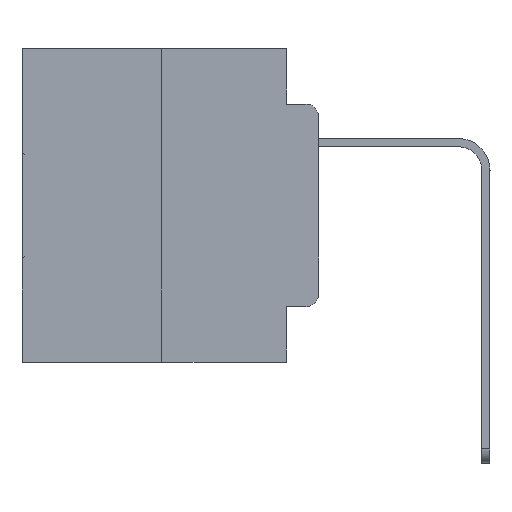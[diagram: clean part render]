
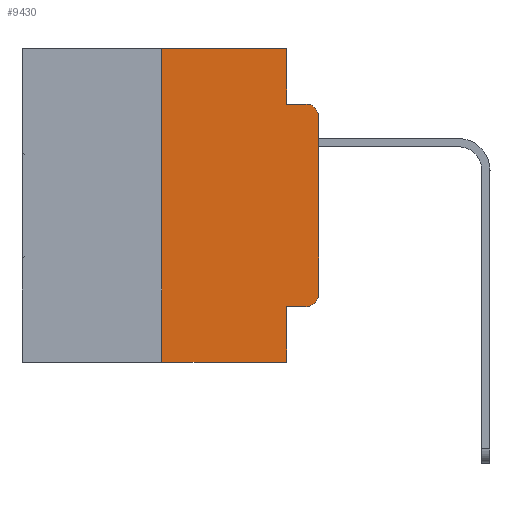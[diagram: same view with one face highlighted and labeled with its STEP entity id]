
A CAD part, left-side view. The second image highlights one B-rep face of the part: STEP entity #9430.
In plain terms, the highlighted planar face has unit normal (-1, 0, 0).
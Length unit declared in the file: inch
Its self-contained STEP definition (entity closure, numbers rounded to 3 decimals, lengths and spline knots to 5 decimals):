
#327 = ORIENTED_EDGE ( 'NONE', *, *, #11311, .F. ) ;
#585 = VECTOR ( 'NONE', #4701, 39.37008 ) ;
#1682 = CARTESIAN_POINT ( 'NONE',  ( 0., 0.473, -0.5 ) ) ;
#2079 = VERTEX_POINT ( 'NONE', #15576 ) ;
#2305 = VERTEX_POINT ( 'NONE', #29038 ) ;
#2365 = VERTEX_POINT ( 'NONE', #29349 ) ;
#2537 = AXIS2_PLACEMENT_3D ( 'NONE', #15377, #6257, #22660 ) ;
#2691 = CARTESIAN_POINT ( 'NONE',  ( 0., 0.473, 0. ) ) ;
#2839 = VERTEX_POINT ( 'NONE', #21788 ) ;
#3406 = CARTESIAN_POINT ( 'NONE',  ( 0., 0.02, -0.0885 ) ) ;
#3701 = DIRECTION ( 'NONE',  ( 0., 0., -1. ) ) ;
#3715 = CARTESIAN_POINT ( 'NONE',  ( 0., 0.25, 0. ) ) ;
#3877 = DIRECTION ( 'NONE',  ( 0., -1., 0. ) ) ;
#4158 = VERTEX_POINT ( 'NONE', #3406 ) ;
#4701 = DIRECTION ( 'NONE',  ( 0., -1., 0. ) ) ;
#4945 = ORIENTED_EDGE ( 'NONE', *, *, #18878, .F. ) ;
#5055 = CARTESIAN_POINT ( 'NONE',  ( 0., 0.25, 0. ) ) ;
#5182 = EDGE_CURVE ( 'NONE', #2079, #2305, #6317, .T. ) ;
#5239 = CARTESIAN_POINT ( 'NONE',  ( 0., 0.02, -0.4115 ) ) ;
#5759 = DIRECTION ( 'NONE',  ( 0., 0., 1. ) ) ;
#6077 = CARTESIAN_POINT ( 'NONE',  ( 0., 0., -0.3915 ) ) ;
#6252 = ORIENTED_EDGE ( 'NONE', *, *, #16830, .T. ) ;
#6257 = DIRECTION ( 'NONE',  ( -1., 0., 0. ) ) ;
#6317 = LINE ( 'NONE', #1682, #27460 ) ;
#6587 = CIRCLE ( 'NONE', #26185, 0.02 ) ;
#6698 = VECTOR ( 'NONE', #26611, 39.37008 ) ;
#6733 = CARTESIAN_POINT ( 'NONE',  ( 0., 0., -0.1085 ) ) ;
#6937 = EDGE_CURVE ( 'NONE', #30050, #4158, #6587, .T. ) ;
#6958 = CARTESIAN_POINT ( 'NONE',  ( 0., 0.051, -0.0885 ) ) ;
#7963 = VERTEX_POINT ( 'NONE', #6077 ) ;
#8077 = VECTOR ( 'NONE', #15972, 39.37008 ) ;
#8496 = DIRECTION ( 'NONE',  ( 0., -1., 0. ) ) ;
#8621 = CARTESIAN_POINT ( 'NONE',  ( 0., 0.051, 0. ) ) ;
#9209 = CIRCLE ( 'NONE', #2537, 0.02 ) ;
#9430 = ADVANCED_FACE ( 'NONE', ( #28254 ), #13706, .F. ) ;
#10420 = ORIENTED_EDGE ( 'NONE', *, *, #19711, .F. ) ;
#10992 = CARTESIAN_POINT ( 'NONE',  ( 0., 0.051, 0. ) ) ;
#11311 = EDGE_CURVE ( 'NONE', #19576, #2839, #13988, .T. ) ;
#12077 = DIRECTION ( 'NONE',  ( -1., 0., 0. ) ) ;
#12873 = EDGE_LOOP ( 'NONE', ( #19832, #13245, #4945, #327, #10420, #28943, #20684, #27754, #17325, #6252 ) ) ;
#12938 = CARTESIAN_POINT ( 'NONE',  ( 0., 0.473, 0. ) ) ;
#13137 = LINE ( 'NONE', #17008, #15370 ) ;
#13245 = ORIENTED_EDGE ( 'NONE', *, *, #6937, .T. ) ;
#13706 = PLANE ( 'NONE',  #25809 ) ;
#13988 = LINE ( 'NONE', #8621, #8077 ) ;
#14831 = VERTEX_POINT ( 'NONE', #5055 ) ;
#15370 = VECTOR ( 'NONE', #24074, 39.37008 ) ;
#15377 = CARTESIAN_POINT ( 'NONE',  ( 0., 0.02, -0.3915 ) ) ;
#15385 = DIRECTION ( 'NONE',  ( 1., 0., 0. ) ) ;
#15576 = CARTESIAN_POINT ( 'NONE',  ( 0., 0.25, -0.5 ) ) ;
#15972 = DIRECTION ( 'NONE',  ( 0., 0., -1. ) ) ;
#16830 = EDGE_CURVE ( 'NONE', #23137, #7963, #9209, .T. ) ;
#17008 = CARTESIAN_POINT ( 'NONE',  ( 0., 0., 0. ) ) ;
#17325 = ORIENTED_EDGE ( 'NONE', *, *, #29895, .T. ) ;
#18878 = EDGE_CURVE ( 'NONE', #2839, #4158, #29069, .T. ) ;
#19039 = EDGE_CURVE ( 'NONE', #7963, #30050, #13137, .T. ) ;
#19576 = VERTEX_POINT ( 'NONE', #21236 ) ;
#19711 = EDGE_CURVE ( 'NONE', #14831, #19576, #27097, .T. ) ;
#19832 = ORIENTED_EDGE ( 'NONE', *, *, #19039, .T. ) ;
#20684 = ORIENTED_EDGE ( 'NONE', *, *, #5182, .T. ) ;
#21236 = CARTESIAN_POINT ( 'NONE',  ( 0., 0.051, 0. ) ) ;
#21339 = EDGE_CURVE ( 'NONE', #2079, #14831, #26990, .T. ) ;
#21788 = CARTESIAN_POINT ( 'NONE',  ( 0., 0.051, -0.0885 ) ) ;
#22129 = EDGE_CURVE ( 'NONE', #2365, #2305, #25481, .T. ) ;
#22660 = DIRECTION ( 'NONE',  ( 0., 0., -1. ) ) ;
#23137 = VERTEX_POINT ( 'NONE', #5239 ) ;
#23936 = CARTESIAN_POINT ( 'NONE',  ( 0., 0.02, -0.1085 ) ) ;
#24074 = DIRECTION ( 'NONE',  ( 0., 0., 1. ) ) ;
#25481 = LINE ( 'NONE', #10992, #27312 ) ;
#25809 = AXIS2_PLACEMENT_3D ( 'NONE', #12938, #15385, #3701 ) ;
#26185 = AXIS2_PLACEMENT_3D ( 'NONE', #23936, #12077, #28644 ) ;
#26611 = DIRECTION ( 'NONE',  ( 0., -1., 0. ) ) ;
#26990 = LINE ( 'NONE', #3715, #30681 ) ;
#27097 = LINE ( 'NONE', #2691, #6698 ) ;
#27312 = VECTOR ( 'NONE', #27681, 39.37008 ) ;
#27460 = VECTOR ( 'NONE', #8496, 39.37008 ) ;
#27681 = DIRECTION ( 'NONE',  ( 0., 0., -1. ) ) ;
#27754 = ORIENTED_EDGE ( 'NONE', *, *, #22129, .F. ) ;
#28254 = FACE_OUTER_BOUND ( 'NONE', #12873, .T. ) ;
#28644 = DIRECTION ( 'NONE',  ( 0., 0., -1. ) ) ;
#28943 = ORIENTED_EDGE ( 'NONE', *, *, #21339, .F. ) ;
#29038 = CARTESIAN_POINT ( 'NONE',  ( 0., 0.051, -0.5 ) ) ;
#29069 = LINE ( 'NONE', #6958, #585 ) ;
#29137 = VECTOR ( 'NONE', #3877, 39.37008 ) ;
#29349 = CARTESIAN_POINT ( 'NONE',  ( 0., 0.051, -0.4115 ) ) ;
#29895 = EDGE_CURVE ( 'NONE', #2365, #23137, #29898, .T. ) ;
#29898 = LINE ( 'NONE', #29939, #29137 ) ;
#29939 = CARTESIAN_POINT ( 'NONE',  ( 0., 0.051, -0.4115 ) ) ;
#30050 = VERTEX_POINT ( 'NONE', #6733 ) ;
#30681 = VECTOR ( 'NONE', #5759, 39.37008 ) ;
